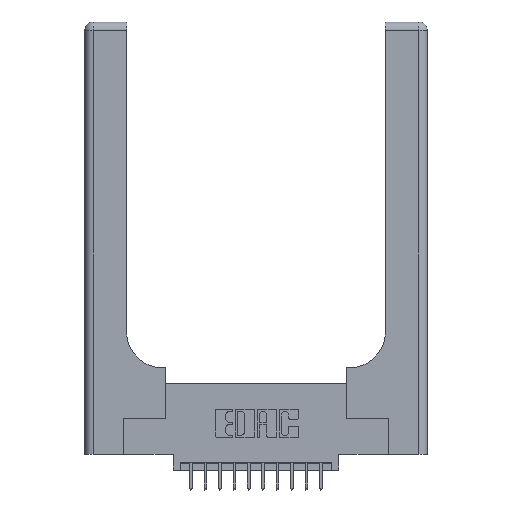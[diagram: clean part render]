
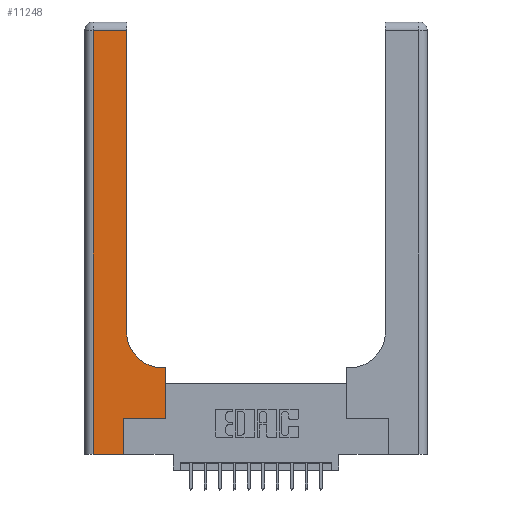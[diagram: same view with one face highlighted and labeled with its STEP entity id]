
A CAD part, top view. The second image highlights one B-rep face of the part: STEP entity #11248.
In plain terms, the highlighted planar face has unit normal (0, 0, 1).
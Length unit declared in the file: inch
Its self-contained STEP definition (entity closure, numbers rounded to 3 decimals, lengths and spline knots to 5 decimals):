
#260 = EDGE_CURVE ( 'NONE', #5664, #4967, #3954, .T. ) ;
#631 = VECTOR ( 'NONE', #7710, 39.37008 ) ;
#774 = CARTESIAN_POINT ( 'NONE',  ( 0.2915, 0.85, 0.37 ) ) ;
#1009 = VECTOR ( 'NONE', #15310, 39.37008 ) ;
#1056 = VERTEX_POINT ( 'NONE', #3617 ) ;
#1700 = EDGE_CURVE ( 'NONE', #15089, #15698, #3398, .T. ) ;
#1816 = CARTESIAN_POINT ( 'NONE',  ( 0.269, 0., 0.37 ) ) ;
#1859 = AXIS2_PLACEMENT_3D ( 'NONE', #14321, #2079, #12995 ) ;
#1933 = EDGE_CURVE ( 'NONE', #1056, #8814, #10430, .T. ) ;
#2079 = DIRECTION ( 'NONE',  ( 0., 0., -1. ) ) ;
#2887 = DIRECTION ( 'NONE',  ( 1., 0., 0. ) ) ;
#3398 = CIRCLE ( 'NONE', #15628, 0.25 ) ;
#3507 = DIRECTION ( 'NONE',  ( 0., 1., 0. ) ) ;
#3617 = CARTESIAN_POINT ( 'NONE',  ( 0.2915, 2.94, 0.37 ) ) ;
#3954 = LINE ( 'NONE', #7017, #8360 ) ;
#4058 = ORIENTED_EDGE ( 'NONE', *, *, #16735, .T. ) ;
#4629 = VECTOR ( 'NONE', #11219, 39.37008 ) ;
#4636 = CARTESIAN_POINT ( 'NONE',  ( 0.2915, 0.6, 0.37 ) ) ;
#4967 = VERTEX_POINT ( 'NONE', #1816 ) ;
#5029 = CARTESIAN_POINT ( 'NONE',  ( 0.5415, 0.6, 0.37 ) ) ;
#5109 = CARTESIAN_POINT ( 'NONE',  ( 0.5585, 0.6, 0.37 ) ) ;
#5664 = VERTEX_POINT ( 'NONE', #12757 ) ;
#5767 = CARTESIAN_POINT ( 'NONE',  ( 0.269, 0.25, 0.37 ) ) ;
#5909 = LINE ( 'NONE', #4636, #631 ) ;
#6266 = LINE ( 'NONE', #15944, #15785 ) ;
#6411 = EDGE_CURVE ( 'NONE', #15176, #15089, #5909, .T. ) ;
#6506 = ORIENTED_EDGE ( 'NONE', *, *, #260, .T. ) ;
#7017 = CARTESIAN_POINT ( 'NONE',  ( 0., 0., 0.37 ) ) ;
#7313 = LINE ( 'NONE', #5767, #4629 ) ;
#7373 = ORIENTED_EDGE ( 'NONE', *, *, #1700, .T. ) ;
#7629 = DIRECTION ( 'NONE',  ( 0., -1., 0. ) ) ;
#7710 = DIRECTION ( 'NONE',  ( -1., 0., 0. ) ) ;
#7959 = DIRECTION ( 'NONE',  ( 0., 0., -1. ) ) ;
#7986 = VECTOR ( 'NONE', #17061, 39.37008 ) ;
#8080 = LINE ( 'NONE', #13493, #16356 ) ;
#8216 = ORIENTED_EDGE ( 'NONE', *, *, #9819, .T. ) ;
#8360 = VECTOR ( 'NONE', #2887, 39.37008 ) ;
#8489 = EDGE_CURVE ( 'NONE', #13069, #10176, #7313, .T. ) ;
#8814 = VERTEX_POINT ( 'NONE', #9128 ) ;
#9128 = CARTESIAN_POINT ( 'NONE',  ( 0.06, 2.94, 0.37 ) ) ;
#9735 = LINE ( 'NONE', #12507, #1009 ) ;
#9819 = EDGE_CURVE ( 'NONE', #4967, #13069, #9735, .T. ) ;
#10176 = VERTEX_POINT ( 'NONE', #14568 ) ;
#10254 = ORIENTED_EDGE ( 'NONE', *, *, #8489, .T. ) ;
#10430 = LINE ( 'NONE', #15729, #7986 ) ;
#10516 = EDGE_CURVE ( 'NONE', #8814, #5664, #6266, .T. ) ;
#10668 = FACE_OUTER_BOUND ( 'NONE', #11457, .T. ) ;
#10911 = DIRECTION ( 'NONE',  ( 0., 1., 0. ) ) ;
#10991 = ORIENTED_EDGE ( 'NONE', *, *, #6411, .T. ) ;
#11219 = DIRECTION ( 'NONE',  ( 1., 0., 0. ) ) ;
#11248 = ADVANCED_FACE ( 'NONE', ( #10668 ), #16059, .F. ) ;
#11457 = EDGE_LOOP ( 'NONE', ( #12798, #13548, #11901, #6506, #8216, #10254, #4058, #10991, #7373 ) ) ;
#11901 = ORIENTED_EDGE ( 'NONE', *, *, #10516, .T. ) ;
#12302 = DIRECTION ( 'NONE',  ( 1., 0., 0. ) ) ;
#12507 = CARTESIAN_POINT ( 'NONE',  ( 0.269, 0., 0.37 ) ) ;
#12697 = VECTOR ( 'NONE', #3507, 39.37008 ) ;
#12757 = CARTESIAN_POINT ( 'NONE',  ( 0.06, 0., 0.37 ) ) ;
#12798 = ORIENTED_EDGE ( 'NONE', *, *, #16838, .T. ) ;
#12995 = DIRECTION ( 'NONE',  ( -1., 0., 0. ) ) ;
#13069 = VERTEX_POINT ( 'NONE', #13791 ) ;
#13493 = CARTESIAN_POINT ( 'NONE',  ( 0.2915, 3., 0.37 ) ) ;
#13548 = ORIENTED_EDGE ( 'NONE', *, *, #1933, .T. ) ;
#13791 = CARTESIAN_POINT ( 'NONE',  ( 0.269, 0.25, 0.37 ) ) ;
#14321 = CARTESIAN_POINT ( 'NONE',  ( 0., 3., 0.37 ) ) ;
#14568 = CARTESIAN_POINT ( 'NONE',  ( 0.5585, 0.25, 0.37 ) ) ;
#14737 = CARTESIAN_POINT ( 'NONE',  ( 0.5585, 0.25, 0.37 ) ) ;
#15089 = VERTEX_POINT ( 'NONE', #5029 ) ;
#15176 = VERTEX_POINT ( 'NONE', #5109 ) ;
#15310 = DIRECTION ( 'NONE',  ( 0., 1., 0. ) ) ;
#15628 = AXIS2_PLACEMENT_3D ( 'NONE', #15926, #7959, #12302 ) ;
#15698 = VERTEX_POINT ( 'NONE', #774 ) ;
#15729 = CARTESIAN_POINT ( 'NONE',  ( 0., 2.94, 0.37 ) ) ;
#15785 = VECTOR ( 'NONE', #7629, 39.37008 ) ;
#15926 = CARTESIAN_POINT ( 'NONE',  ( 0.5415, 0.85, 0.37 ) ) ;
#15944 = CARTESIAN_POINT ( 'NONE',  ( 0.06, 3., 0.37 ) ) ;
#16059 = PLANE ( 'NONE',  #1859 ) ;
#16356 = VECTOR ( 'NONE', #10911, 39.37008 ) ;
#16735 = EDGE_CURVE ( 'NONE', #10176, #15176, #17214, .T. ) ;
#16838 = EDGE_CURVE ( 'NONE', #15698, #1056, #8080, .T. ) ;
#17061 = DIRECTION ( 'NONE',  ( -1., 0., 0. ) ) ;
#17214 = LINE ( 'NONE', #14737, #12697 ) ;
